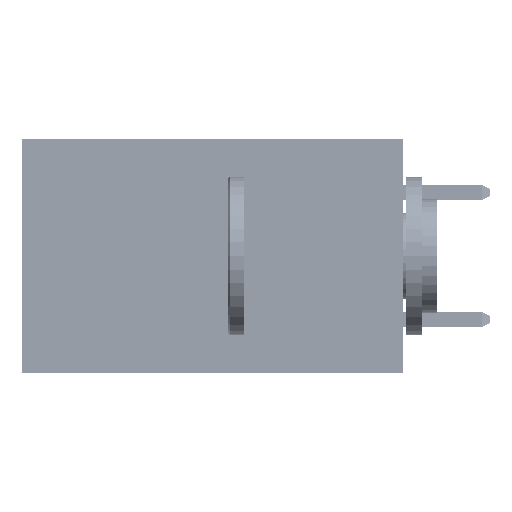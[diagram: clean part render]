
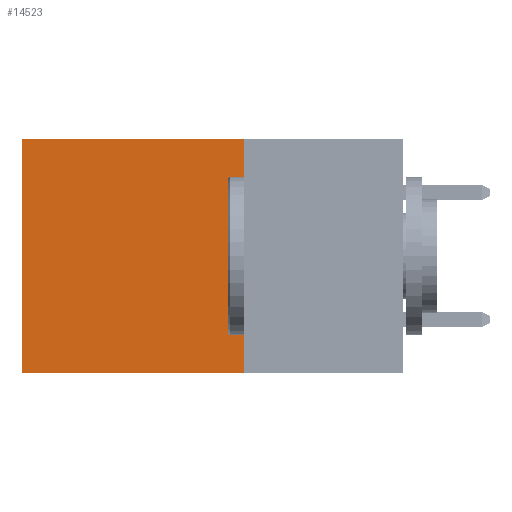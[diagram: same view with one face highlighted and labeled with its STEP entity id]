
A CAD part, left-side view. The second image highlights one B-rep face of the part: STEP entity #14523.
In plain terms, the highlighted planar face has unit normal (-1, 0, 0).
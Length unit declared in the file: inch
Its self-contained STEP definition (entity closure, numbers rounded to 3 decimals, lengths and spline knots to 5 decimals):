
#82 = EDGE_CURVE ( 'NONE', #17282, #50307, #10074, .T. ) ;
#3069 = CARTESIAN_POINT ( 'NONE',  ( 0.2875, 0.6, -0.37 ) ) ;
#3198 = DIRECTION ( 'NONE',  ( 0., 0., -1. ) ) ;
#4670 = VECTOR ( 'NONE', #14837, 39.37008 ) ;
#5286 = CARTESIAN_POINT ( 'NONE',  ( 0.2875, 0.25, 0. ) ) ;
#5381 = VERTEX_POINT ( 'NONE', #51390 ) ;
#5523 = ORIENTED_EDGE ( 'NONE', *, *, #13446, .F. ) ;
#6914 = CARTESIAN_POINT ( 'NONE',  ( 0.2875, 0.25, 0. ) ) ;
#8369 = EDGE_CURVE ( 'NONE', #5381, #42741, #27997, .T. ) ;
#9706 = LINE ( 'NONE', #32856, #20534 ) ;
#10074 = LINE ( 'NONE', #5286, #29781 ) ;
#13446 = EDGE_CURVE ( 'NONE', #50307, #42741, #9706, .T. ) ;
#14523 = ADVANCED_FACE ( 'NONE', ( #26118 ), #31196, .F. ) ;
#14837 = DIRECTION ( 'NONE',  ( 0., 1., 0. ) ) ;
#17282 = VERTEX_POINT ( 'NONE', #39480 ) ;
#18584 = EDGE_CURVE ( 'NONE', #17282, #5381, #37059, .T. ) ;
#20534 = VECTOR ( 'NONE', #48811, 39.37008 ) ;
#24491 = ORIENTED_EDGE ( 'NONE', *, *, #18584, .T. ) ;
#26118 = FACE_OUTER_BOUND ( 'NONE', #49814, .T. ) ;
#26864 = DIRECTION ( 'NONE',  ( 0., 0., -1. ) ) ;
#27997 = LINE ( 'NONE', #39617, #42589 ) ;
#29768 = ORIENTED_EDGE ( 'NONE', *, *, #8369, .T. ) ;
#29781 = VECTOR ( 'NONE', #3198, 39.37008 ) ;
#30596 = CARTESIAN_POINT ( 'NONE',  ( 0.2875, 0.25, 0. ) ) ;
#31196 = PLANE ( 'NONE',  #35571 ) ;
#31642 = CARTESIAN_POINT ( 'NONE',  ( 0.2875, 0.25, -0.37 ) ) ;
#32856 = CARTESIAN_POINT ( 'NONE',  ( 0.2875, 0.25, -0.37 ) ) ;
#35275 = DIRECTION ( 'NONE',  ( 1., 0., 0. ) ) ;
#35571 = AXIS2_PLACEMENT_3D ( 'NONE', #6914, #35275, #39353 ) ;
#37059 = LINE ( 'NONE', #30596, #4670 ) ;
#39353 = DIRECTION ( 'NONE',  ( 0., 0., -1. ) ) ;
#39480 = CARTESIAN_POINT ( 'NONE',  ( 0.2875, 0.25, 0. ) ) ;
#39617 = CARTESIAN_POINT ( 'NONE',  ( 0.2875, 0.6, 0. ) ) ;
#42589 = VECTOR ( 'NONE', #26864, 39.37008 ) ;
#42741 = VERTEX_POINT ( 'NONE', #3069 ) ;
#48020 = ORIENTED_EDGE ( 'NONE', *, *, #82, .F. ) ;
#48811 = DIRECTION ( 'NONE',  ( 0., 1., 0. ) ) ;
#49814 = EDGE_LOOP ( 'NONE', ( #29768, #5523, #48020, #24491 ) ) ;
#50307 = VERTEX_POINT ( 'NONE', #31642 ) ;
#51390 = CARTESIAN_POINT ( 'NONE',  ( 0.2875, 0.6, 0. ) ) ;
